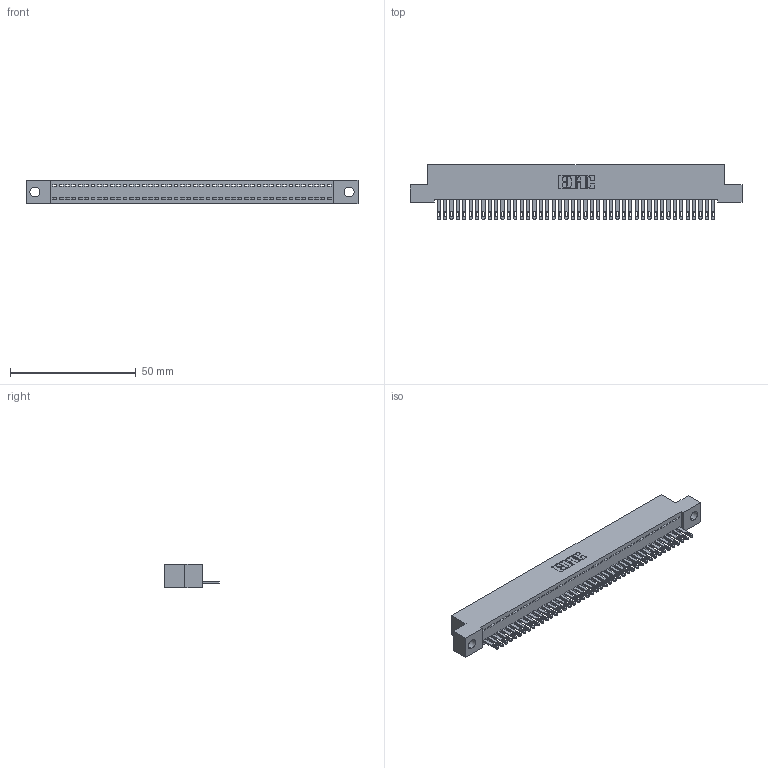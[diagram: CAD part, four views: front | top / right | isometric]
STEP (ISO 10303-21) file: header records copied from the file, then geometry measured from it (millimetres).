
FILE_DESCRIPTION (( 'STEP AP203' ), '1' );
FILE_NAME ('342-044-500-104.STEP', '2018-08-12T14:07:58', ( '' ), ( '' ), 'SwSTEP 2.0', 'SolidWorks 2016', '' );
FILE_SCHEMA (( 'CONFIG_CONTROL_DESIGN' ));
Length unit declared in the file: inch
Products named in the file (3): 342 Part_.156 TH; 345-292-001_345-293-100; 342-044-500-104
Assembly tree (45 placements, depth 2):
  342-044-500-104
    342 Part_.156 TH
    345-292-001_345-293-100  x44
Bounding box: 132.08 x 21.85 x 9.4 mm (x, y, z)
Volume: 11528.4 mm3; surface area: 16871.6 mm2
Topology: 45 solids, 45 shells, 2486 faces, 7691 edges, 5126 vertices
Faces by surface type: plane 1650, cylinder 836
Entity records: 26441 total; most frequent: CARTESIAN_POINT 4566, ORIENTED_EDGE 4546, DIRECTION 3849, EDGE_CURVE 2273, VECTOR 2141, LINE 2141, VERTEX_POINT 1514, AXIS2_PLACEMENT_3D 854
